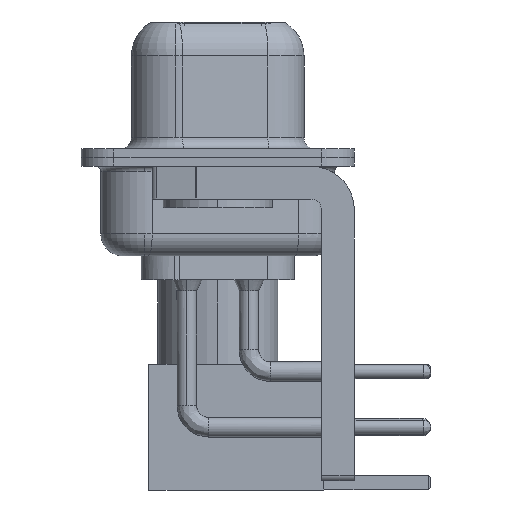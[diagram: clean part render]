
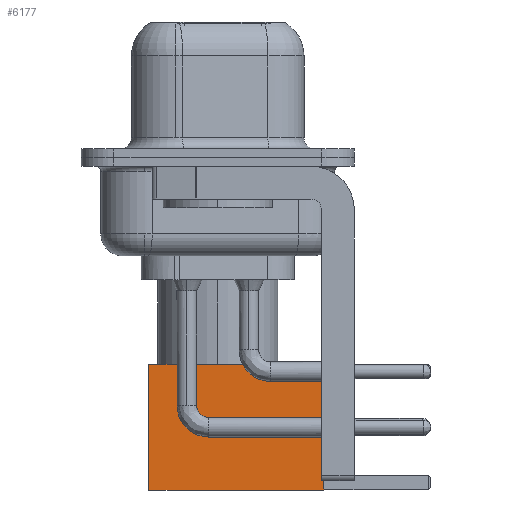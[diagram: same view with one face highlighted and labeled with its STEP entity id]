
A CAD part, left-side view. The second image highlights one B-rep face of the part: STEP entity #6177.
In plain terms, the highlighted face is planar.
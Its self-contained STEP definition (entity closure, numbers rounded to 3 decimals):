
#255 = CARTESIAN_POINT ( 'NONE',  ( 2.875, 2.875, 0. ) ) ;
#362 = EDGE_CURVE ( 'NONE', #11504, #11320, #5406, .T. ) ;
#594 = VECTOR ( 'NONE', #5579, 1000. ) ;
#789 = CARTESIAN_POINT ( 'NONE',  ( 2.875, 2.875, 0. ) ) ;
#2217 = AXIS2_PLACEMENT_3D ( 'NONE', #2479, #6975, #5267 ) ;
#2479 = CARTESIAN_POINT ( 'NONE',  ( 2.875, 2.875, 0. ) ) ;
#2498 = ORIENTED_EDGE ( 'NONE', *, *, #362, .T. ) ;
#3759 = VERTEX_POINT ( 'NONE', #13158 ) ;
#3766 = DIRECTION ( 'NONE',  ( 0., 0., -1. ) ) ;
#4041 = CARTESIAN_POINT ( 'NONE',  ( 0., 2.875, 8. ) ) ;
#5267 = DIRECTION ( 'NONE',  ( 0., 0., 1. ) ) ;
#5406 = LINE ( 'NONE', #789, #8119 ) ;
#5579 = DIRECTION ( 'NONE',  ( -1., 0., 0. ) ) ;
#6153 = EDGE_CURVE ( 'NONE', #11320, #3759, #8708, .T. ) ;
#6177 = ADVANCED_FACE ( 'NONE', ( #11667 ), #17704, .T. ) ;
#6975 = DIRECTION ( 'NONE',  ( 0., 1., 0. ) ) ;
#8119 = VECTOR ( 'NONE', #3766, 1000. ) ;
#8228 = CARTESIAN_POINT ( 'NONE',  ( -2.875, 2.875, 8. ) ) ;
#8490 = VECTOR ( 'NONE', #18026, 1000. ) ;
#8708 = LINE ( 'NONE', #14751, #594 ) ;
#10068 = DIRECTION ( 'NONE',  ( 0., 0., -1. ) ) ;
#10599 = VERTEX_POINT ( 'NONE', #8228 ) ;
#10775 = ORIENTED_EDGE ( 'NONE', *, *, #6153, .T. ) ;
#11320 = VERTEX_POINT ( 'NONE', #255 ) ;
#11504 = VERTEX_POINT ( 'NONE', #13012 ) ;
#11667 = FACE_OUTER_BOUND ( 'NONE', #14568, .T. ) ;
#11702 = CARTESIAN_POINT ( 'NONE',  ( -2.875, 2.875, 0. ) ) ;
#11998 = VECTOR ( 'NONE', #10068, 1000. ) ;
#13012 = CARTESIAN_POINT ( 'NONE',  ( 2.875, 2.875, 8. ) ) ;
#13112 = EDGE_CURVE ( 'NONE', #10599, #3759, #17844, .T. ) ;
#13158 = CARTESIAN_POINT ( 'NONE',  ( -2.875, 2.875, 0. ) ) ;
#14568 = EDGE_LOOP ( 'NONE', ( #2498, #10775, #18654, #17052 ) ) ;
#14751 = CARTESIAN_POINT ( 'NONE',  ( 0., 2.875, 0. ) ) ;
#15221 = EDGE_CURVE ( 'NONE', #11504, #10599, #18124, .T. ) ;
#17052 = ORIENTED_EDGE ( 'NONE', *, *, #15221, .F. ) ;
#17704 = PLANE ( 'NONE',  #2217 ) ;
#17844 = LINE ( 'NONE', #11702, #11998 ) ;
#18026 = DIRECTION ( 'NONE',  ( -1., 0., 0. ) ) ;
#18124 = LINE ( 'NONE', #4041, #8490 ) ;
#18654 = ORIENTED_EDGE ( 'NONE', *, *, #13112, .F. ) ;
